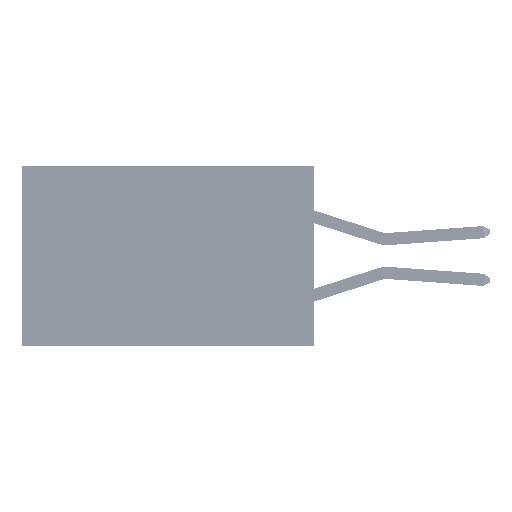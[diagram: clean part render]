
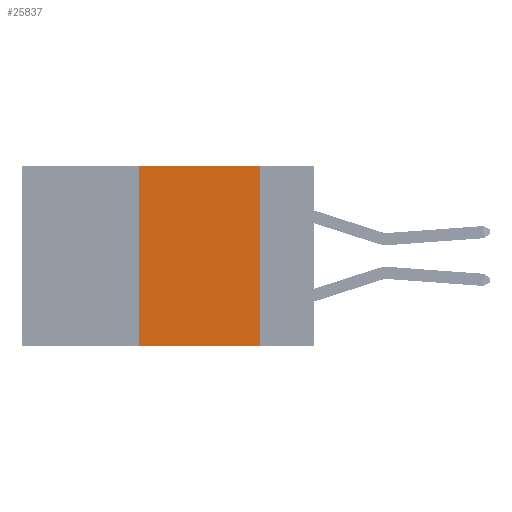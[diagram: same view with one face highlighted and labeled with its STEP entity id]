
A CAD part, left-side view. The second image highlights one B-rep face of the part: STEP entity #25837.
In plain terms, the highlighted planar face has unit normal (-1, 0, 0).
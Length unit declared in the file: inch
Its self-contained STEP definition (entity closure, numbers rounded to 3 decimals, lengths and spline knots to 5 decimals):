
#219 = ORIENTED_EDGE ( 'NONE', *, *, #13628, .F. ) ;
#478 = CARTESIAN_POINT ( 'NONE',  ( 0., 0.6, 0. ) ) ;
#2059 = DIRECTION ( 'NONE',  ( 0., 0., -1. ) ) ;
#2594 = EDGE_CURVE ( 'NONE', #8224, #48840, #29675, .T. ) ;
#6374 = VERTEX_POINT ( 'NONE', #30124 ) ;
#8224 = VERTEX_POINT ( 'NONE', #10313 ) ;
#9483 = AXIS2_PLACEMENT_3D ( 'NONE', #43332, #28031, #31908 ) ;
#9532 = CARTESIAN_POINT ( 'NONE',  ( 0., 0.11, 0. ) ) ;
#10313 = CARTESIAN_POINT ( 'NONE',  ( 0., 0.36, -0.37 ) ) ;
#11275 = CARTESIAN_POINT ( 'NONE',  ( 0., 0.6, -0.37 ) ) ;
#12198 = LINE ( 'NONE', #41753, #41815 ) ;
#12564 = DIRECTION ( 'NONE',  ( 0., -1., 0. ) ) ;
#13378 = EDGE_LOOP ( 'NONE', ( #219, #29015, #28328, #47762 ) ) ;
#13628 = EDGE_CURVE ( 'NONE', #21525, #48840, #16690, .T. ) ;
#14566 = DIRECTION ( 'NONE',  ( 0., 0., 1. ) ) ;
#14723 = CARTESIAN_POINT ( 'NONE',  ( 0., 0.11, -0.37 ) ) ;
#16690 = LINE ( 'NONE', #17358, #43854 ) ;
#17358 = CARTESIAN_POINT ( 'NONE',  ( 0., 0.11, 0. ) ) ;
#20047 = PLANE ( 'NONE',  #9483 ) ;
#20568 = VECTOR ( 'NONE', #38348, 39.37008 ) ;
#21525 = VERTEX_POINT ( 'NONE', #9532 ) ;
#22123 = EDGE_CURVE ( 'NONE', #6374, #21525, #26505, .T. ) ;
#22579 = FACE_OUTER_BOUND ( 'NONE', #13378, .T. ) ;
#25837 = ADVANCED_FACE ( 'NONE', ( #22579 ), #20047, .F. ) ;
#26505 = LINE ( 'NONE', #478, #37376 ) ;
#26940 = EDGE_CURVE ( 'NONE', #8224, #6374, #12198, .T. ) ;
#28031 = DIRECTION ( 'NONE',  ( 1., 0., 0. ) ) ;
#28328 = ORIENTED_EDGE ( 'NONE', *, *, #26940, .F. ) ;
#29015 = ORIENTED_EDGE ( 'NONE', *, *, #22123, .F. ) ;
#29675 = LINE ( 'NONE', #11275, #20568 ) ;
#30124 = CARTESIAN_POINT ( 'NONE',  ( 0., 0.36, 0. ) ) ;
#31908 = DIRECTION ( 'NONE',  ( 0., 0., -1. ) ) ;
#37376 = VECTOR ( 'NONE', #12564, 39.37008 ) ;
#38348 = DIRECTION ( 'NONE',  ( 0., -1., 0. ) ) ;
#41753 = CARTESIAN_POINT ( 'NONE',  ( 0., 0.36, 0. ) ) ;
#41815 = VECTOR ( 'NONE', #14566, 39.37008 ) ;
#43332 = CARTESIAN_POINT ( 'NONE',  ( 0., 0.6, 0. ) ) ;
#43854 = VECTOR ( 'NONE', #2059, 39.37008 ) ;
#47762 = ORIENTED_EDGE ( 'NONE', *, *, #2594, .T. ) ;
#48840 = VERTEX_POINT ( 'NONE', #14723 ) ;
